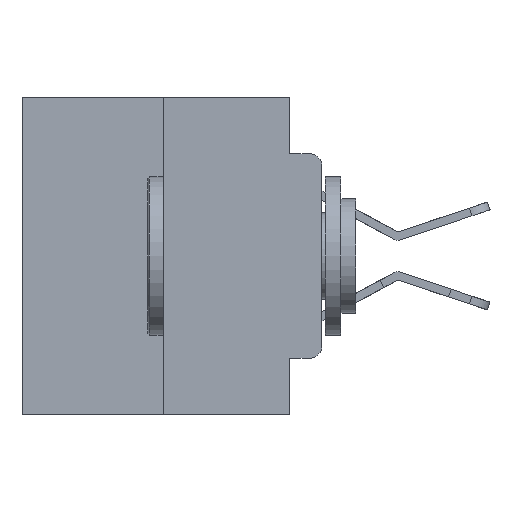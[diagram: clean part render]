
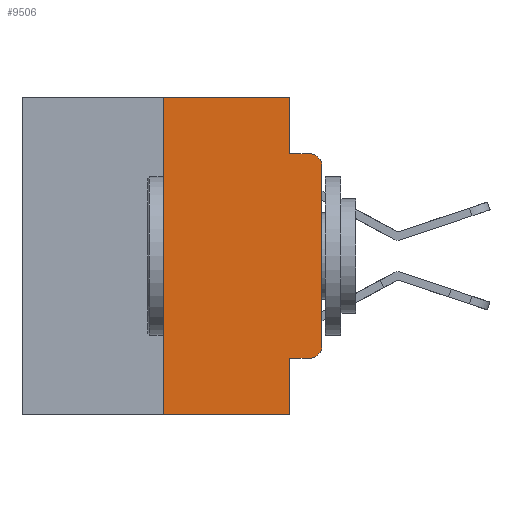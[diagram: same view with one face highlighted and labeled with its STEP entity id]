
A CAD part, left-side view. The second image highlights one B-rep face of the part: STEP entity #9506.
In plain terms, the highlighted planar face has unit normal (-1, 0, 0).
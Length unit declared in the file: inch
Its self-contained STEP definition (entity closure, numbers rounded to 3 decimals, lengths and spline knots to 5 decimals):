
#380 = LINE ( 'NONE', #8699, #11229 ) ;
#516 = DIRECTION ( 'NONE',  ( 0., 0., 1. ) ) ;
#2336 = CARTESIAN_POINT ( 'NONE',  ( 0., 0.051, -0.4115 ) ) ;
#2533 = VECTOR ( 'NONE', #7075, 39.37008 ) ;
#2635 = CARTESIAN_POINT ( 'NONE',  ( 0., 0., 0. ) ) ;
#3028 = VECTOR ( 'NONE', #4589, 39.37008 ) ;
#3216 = DIRECTION ( 'NONE',  ( 0., -1., 0. ) ) ;
#3762 = LINE ( 'NONE', #2336, #3028 ) ;
#3877 = LINE ( 'NONE', #15502, #19577 ) ;
#4062 = CARTESIAN_POINT ( 'NONE',  ( 0., 0.051, -0.0885 ) ) ;
#4589 = DIRECTION ( 'NONE',  ( 0., -1., 0. ) ) ;
#4894 = CARTESIAN_POINT ( 'NONE',  ( 0., 0.051, 0. ) ) ;
#4952 = VERTEX_POINT ( 'NONE', #12945 ) ;
#5120 = ORIENTED_EDGE ( 'NONE', *, *, #11142, .T. ) ;
#5394 = ORIENTED_EDGE ( 'NONE', *, *, #23455, .T. ) ;
#5697 = ORIENTED_EDGE ( 'NONE', *, *, #5881, .F. ) ;
#5825 = VERTEX_POINT ( 'NONE', #17916 ) ;
#5881 = EDGE_CURVE ( 'NONE', #20128, #6681, #18732, .T. ) ;
#6113 = PLANE ( 'NONE',  #18159 ) ;
#6335 = ORIENTED_EDGE ( 'NONE', *, *, #25483, .F. ) ;
#6681 = VERTEX_POINT ( 'NONE', #14379 ) ;
#7074 = DIRECTION ( 'NONE',  ( 0., 0., 1. ) ) ;
#7075 = DIRECTION ( 'NONE',  ( 0., 0., -1. ) ) ;
#7496 = VECTOR ( 'NONE', #7074, 39.37008 ) ;
#7523 = LINE ( 'NONE', #16146, #18442 ) ;
#7788 = VERTEX_POINT ( 'NONE', #8870 ) ;
#8251 = EDGE_CURVE ( 'NONE', #19365, #8547, #9562, .T. ) ;
#8547 = VERTEX_POINT ( 'NONE', #9201 ) ;
#8699 = CARTESIAN_POINT ( 'NONE',  ( 0., 0.473, 0. ) ) ;
#8731 = AXIS2_PLACEMENT_3D ( 'NONE', #11795, #26714, #13927 ) ;
#8870 = CARTESIAN_POINT ( 'NONE',  ( 0., 0.051, -0.4115 ) ) ;
#9201 = CARTESIAN_POINT ( 'NONE',  ( 0., 0.051, -0.5 ) ) ;
#9506 = ADVANCED_FACE ( 'NONE', ( #17533 ), #6113, .F. ) ;
#9562 = LINE ( 'NONE', #18921, #25870 ) ;
#9717 = VERTEX_POINT ( 'NONE', #26061 ) ;
#9731 = DIRECTION ( 'NONE',  ( 0., 0., -1. ) ) ;
#9746 = CIRCLE ( 'NONE', #20754, 0.02 ) ;
#10236 = EDGE_LOOP ( 'NONE', ( #5120, #5394, #5697, #6335, #15966, #17808, #14630, #13703, #12584, #12216 ) ) ;
#11142 = EDGE_CURVE ( 'NONE', #5825, #4952, #18802, .T. ) ;
#11229 = VECTOR ( 'NONE', #25711, 39.37008 ) ;
#11795 = CARTESIAN_POINT ( 'NONE',  ( 0., 0.02, -0.3915 ) ) ;
#12216 = ORIENTED_EDGE ( 'NONE', *, *, #21132, .T. ) ;
#12241 = DIRECTION ( 'NONE',  ( -1., 0., 0. ) ) ;
#12536 = DIRECTION ( 'NONE',  ( 0., 0., -1. ) ) ;
#12584 = ORIENTED_EDGE ( 'NONE', *, *, #13747, .T. ) ;
#12945 = CARTESIAN_POINT ( 'NONE',  ( 0., 0., -0.1085 ) ) ;
#13371 = EDGE_CURVE ( 'NONE', #7788, #8547, #7523, .T. ) ;
#13703 = ORIENTED_EDGE ( 'NONE', *, *, #13371, .F. ) ;
#13747 = EDGE_CURVE ( 'NONE', #7788, #14507, #3762, .T. ) ;
#13927 = DIRECTION ( 'NONE',  ( 0., 0., -1. ) ) ;
#14379 = CARTESIAN_POINT ( 'NONE',  ( 0., 0.02, -0.0885 ) ) ;
#14507 = VERTEX_POINT ( 'NONE', #26129 ) ;
#14630 = ORIENTED_EDGE ( 'NONE', *, *, #8251, .T. ) ;
#15502 = CARTESIAN_POINT ( 'NONE',  ( 0., 0.25, 0. ) ) ;
#15966 = ORIENTED_EDGE ( 'NONE', *, *, #20808, .F. ) ;
#16146 = CARTESIAN_POINT ( 'NONE',  ( 0., 0.051, 0. ) ) ;
#17374 = CARTESIAN_POINT ( 'NONE',  ( 0., 0.051, 0. ) ) ;
#17533 = FACE_OUTER_BOUND ( 'NONE', #10236, .T. ) ;
#17808 = ORIENTED_EDGE ( 'NONE', *, *, #21607, .F. ) ;
#17916 = CARTESIAN_POINT ( 'NONE',  ( 0., 0., -0.3915 ) ) ;
#18159 = AXIS2_PLACEMENT_3D ( 'NONE', #18950, #25316, #12536 ) ;
#18442 = VECTOR ( 'NONE', #9731, 39.37008 ) ;
#18732 = LINE ( 'NONE', #20269, #23649 ) ;
#18802 = LINE ( 'NONE', #2635, #7496 ) ;
#18921 = CARTESIAN_POINT ( 'NONE',  ( 0., 0.473, -0.5 ) ) ;
#18950 = CARTESIAN_POINT ( 'NONE',  ( 0., 0.473, 0. ) ) ;
#19365 = VERTEX_POINT ( 'NONE', #25133 ) ;
#19577 = VECTOR ( 'NONE', #516, 39.37008 ) ;
#19669 = LINE ( 'NONE', #4894, #2533 ) ;
#20128 = VERTEX_POINT ( 'NONE', #4062 ) ;
#20269 = CARTESIAN_POINT ( 'NONE',  ( 0., 0.051, -0.0885 ) ) ;
#20754 = AXIS2_PLACEMENT_3D ( 'NONE', #25027, #12241, #27166 ) ;
#20808 = EDGE_CURVE ( 'NONE', #9717, #23890, #380, .T. ) ;
#20956 = CIRCLE ( 'NONE', #8731, 0.02 ) ;
#21069 = DIRECTION ( 'NONE',  ( 0., -1., 0. ) ) ;
#21132 = EDGE_CURVE ( 'NONE', #14507, #5825, #20956, .T. ) ;
#21607 = EDGE_CURVE ( 'NONE', #19365, #9717, #3877, .T. ) ;
#23455 = EDGE_CURVE ( 'NONE', #4952, #6681, #9746, .T. ) ;
#23649 = VECTOR ( 'NONE', #3216, 39.37008 ) ;
#23890 = VERTEX_POINT ( 'NONE', #17374 ) ;
#25027 = CARTESIAN_POINT ( 'NONE',  ( 0., 0.02, -0.1085 ) ) ;
#25133 = CARTESIAN_POINT ( 'NONE',  ( 0., 0.25, -0.5 ) ) ;
#25316 = DIRECTION ( 'NONE',  ( 1., 0., 0. ) ) ;
#25483 = EDGE_CURVE ( 'NONE', #23890, #20128, #19669, .T. ) ;
#25711 = DIRECTION ( 'NONE',  ( 0., -1., 0. ) ) ;
#25870 = VECTOR ( 'NONE', #21069, 39.37008 ) ;
#26061 = CARTESIAN_POINT ( 'NONE',  ( 0., 0.25, 0. ) ) ;
#26129 = CARTESIAN_POINT ( 'NONE',  ( 0., 0.02, -0.4115 ) ) ;
#26714 = DIRECTION ( 'NONE',  ( -1., 0., 0. ) ) ;
#27166 = DIRECTION ( 'NONE',  ( 0., 0., -1. ) ) ;
